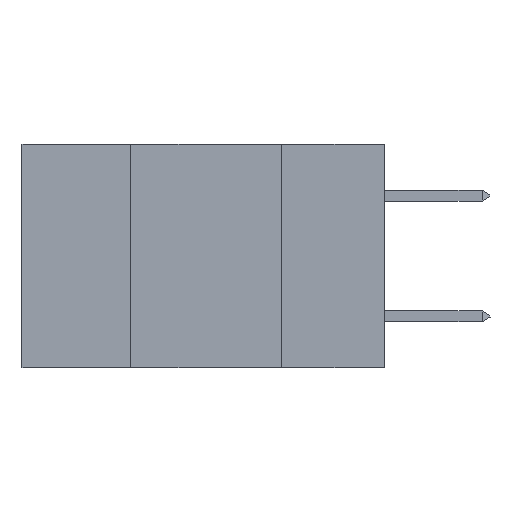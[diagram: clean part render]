
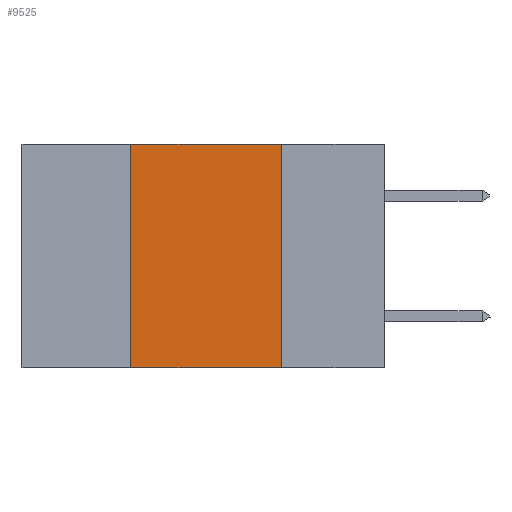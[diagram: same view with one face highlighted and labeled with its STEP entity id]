
A CAD part, left-side view. The second image highlights one B-rep face of the part: STEP entity #9525.
In plain terms, the highlighted planar face has unit normal (-1, 0, 0).
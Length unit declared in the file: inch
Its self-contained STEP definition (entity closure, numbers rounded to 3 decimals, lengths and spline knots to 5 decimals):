
#60 = CARTESIAN_POINT ( 'NONE',  ( 0., 0.6, 0. ) ) ;
#897 = ORIENTED_EDGE ( 'NONE', *, *, #10536, .F. ) ;
#1337 = DIRECTION ( 'NONE',  ( 0., 0., -1. ) ) ;
#1664 = VERTEX_POINT ( 'NONE', #13511 ) ;
#2089 = LINE ( 'NONE', #9008, #3889 ) ;
#2453 = CARTESIAN_POINT ( 'NONE',  ( 0., 0.42, -0.37 ) ) ;
#2863 = EDGE_CURVE ( 'NONE', #11667, #6174, #15319, .T. ) ;
#2914 = ORIENTED_EDGE ( 'NONE', *, *, #14008, .T. ) ;
#3229 = CARTESIAN_POINT ( 'NONE',  ( 0., 0.6, 0. ) ) ;
#3889 = VECTOR ( 'NONE', #10346, 39.37008 ) ;
#5820 = DIRECTION ( 'NONE',  ( 0., -1., 0. ) ) ;
#5893 = CARTESIAN_POINT ( 'NONE',  ( 0., 0.6, -0.37 ) ) ;
#5990 = ORIENTED_EDGE ( 'NONE', *, *, #2863, .F. ) ;
#6174 = VERTEX_POINT ( 'NONE', #15801 ) ;
#7286 = LINE ( 'NONE', #3229, #13468 ) ;
#7479 = AXIS2_PLACEMENT_3D ( 'NONE', #60, #9100, #1337 ) ;
#7903 = CARTESIAN_POINT ( 'NONE',  ( 0., 0.17, 0. ) ) ;
#8265 = CARTESIAN_POINT ( 'NONE',  ( 0., 0.17, 0. ) ) ;
#8756 = EDGE_CURVE ( 'NONE', #15436, #1664, #2089, .T. ) ;
#9008 = CARTESIAN_POINT ( 'NONE',  ( 0., 0.42, 0. ) ) ;
#9100 = DIRECTION ( 'NONE',  ( 1., 0., 0. ) ) ;
#9525 = ADVANCED_FACE ( 'NONE', ( #15125 ), #13023, .F. ) ;
#10346 = DIRECTION ( 'NONE',  ( 0., 0., 1. ) ) ;
#10536 = EDGE_CURVE ( 'NONE', #1664, #11667, #7286, .T. ) ;
#11440 = VECTOR ( 'NONE', #11867, 39.37008 ) ;
#11667 = VERTEX_POINT ( 'NONE', #8265 ) ;
#11725 = VECTOR ( 'NONE', #15065, 39.37008 ) ;
#11867 = DIRECTION ( 'NONE',  ( 0., 0., -1. ) ) ;
#13023 = PLANE ( 'NONE',  #7479 ) ;
#13468 = VECTOR ( 'NONE', #5820, 39.37008 ) ;
#13511 = CARTESIAN_POINT ( 'NONE',  ( 0., 0.42, 0. ) ) ;
#14008 = EDGE_CURVE ( 'NONE', #15436, #6174, #15197, .T. ) ;
#15065 = DIRECTION ( 'NONE',  ( 0., -1., 0. ) ) ;
#15125 = FACE_OUTER_BOUND ( 'NONE', #15154, .T. ) ;
#15154 = EDGE_LOOP ( 'NONE', ( #5990, #897, #15475, #2914 ) ) ;
#15197 = LINE ( 'NONE', #5893, #11725 ) ;
#15319 = LINE ( 'NONE', #7903, #11440 ) ;
#15436 = VERTEX_POINT ( 'NONE', #2453 ) ;
#15475 = ORIENTED_EDGE ( 'NONE', *, *, #8756, .F. ) ;
#15801 = CARTESIAN_POINT ( 'NONE',  ( 0., 0.17, -0.37 ) ) ;
